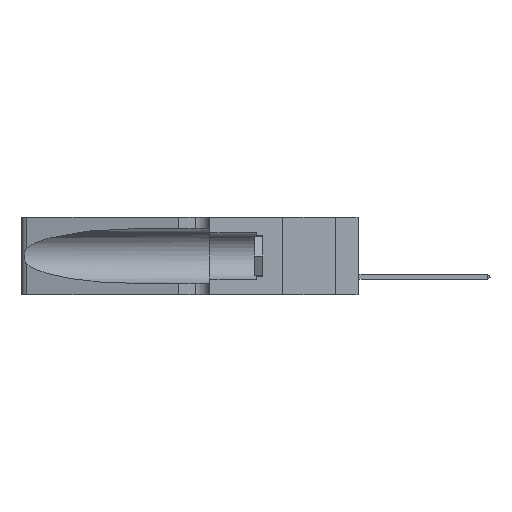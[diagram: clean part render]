
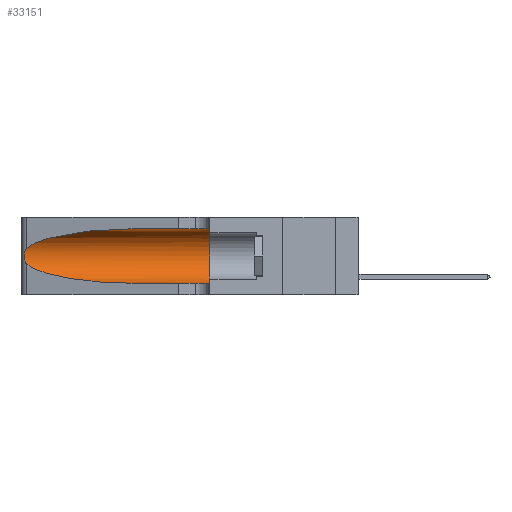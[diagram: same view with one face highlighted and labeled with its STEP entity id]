
A CAD part, left-side view. The second image highlights one B-rep face of the part: STEP entity #33151.
In plain terms, the highlighted cylindrical face has radius 3.308 mm (diameter 6.617 mm), a partial arc.
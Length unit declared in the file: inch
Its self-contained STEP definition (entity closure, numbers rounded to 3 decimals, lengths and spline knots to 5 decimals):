
#1242 = EDGE_CURVE ( 'NONE', #28191, #19521, #26771, .T. ) ;
#3250 = CARTESIAN_POINT ( 'NONE',  ( 0.1305, 0.72297, 0.05475 ) ) ;
#3714 = CARTESIAN_POINT ( 'NONE',  ( 0.25487, 1.22718, 0.14631 ) ) ;
#3749 = CIRCLE ( 'NONE', #8583, 0.13025 ) ;
#3908 = ORIENTED_EDGE ( 'NONE', *, *, #32514, .T. ) ;
#4390 =( BOUNDED_CURVE ( )  B_SPLINE_CURVE ( 3, ( #7320, #26133, #10004, #15291 ),
 .UNSPECIFIED., .F., .T. ) 
 B_SPLINE_CURVE_WITH_KNOTS ( ( 4, 4 ),
 ( 1.5708, 2.84003 ),
 .UNSPECIFIED. ) 
 CURVE ( )  GEOMETRIC_REPRESENTATION_ITEM ( )  RATIONAL_B_SPLINE_CURVE ( ( 1., 0.87, 0.87, 1. ) ) 
 REPRESENTATION_ITEM ( '' )  );
#5244 = EDGE_CURVE ( 'NONE', #26156, #19521, #3749, .T. ) ;
#5554 = VECTOR ( 'NONE', #18479, 39.37008 ) ;
#7320 = CARTESIAN_POINT ( 'NONE',  ( 0.1305, 0.72297, 0.31525 ) ) ;
#7625 = CARTESIAN_POINT ( 'NONE',  ( 0.25856, 1.23593, 0.16098 ) ) ;
#7730 = CARTESIAN_POINT ( 'NONE',  ( 0.25487, 1.22718, 0.14631 ) ) ;
#7751 = AXIS2_PLACEMENT_3D ( 'NONE', #30096, #32806, #21855 ) ;
#7841 = CARTESIAN_POINT ( 'NONE',  ( 0.25787, 1.23484, 0.2124 ) ) ;
#8583 = AXIS2_PLACEMENT_3D ( 'NONE', #32872, #8798, #27880 ) ;
#8798 = DIRECTION ( 'NONE',  ( 0., 1., 0. ) ) ;
#8917 = CARTESIAN_POINT ( 'NONE',  ( 0.1305, 0.72297, 0.31525 ) ) ;
#8945 = CARTESIAN_POINT ( 'NONE',  ( 0.1305, 0.35, 0.05475 ) ) ;
#9864 = VECTOR ( 'NONE', #13923, 39.37008 ) ;
#10004 = CARTESIAN_POINT ( 'NONE',  ( 0.2373, 1.15595, 0.28018 ) ) ;
#10185 = CARTESIAN_POINT ( 'NONE',  ( 0.26075, 1.23896, 0.178 ) ) ;
#10709 = VERTEX_POINT ( 'NONE', #32028 ) ;
#11398 = CARTESIAN_POINT ( 'NONE',  ( 0.25487, 1.22718, 0.14631 ) ) ;
#13778 = VERTEX_POINT ( 'NONE', #3714 ) ;
#13923 = DIRECTION ( 'NONE',  ( 0., -1., 0. ) ) ;
#14568 = ORIENTED_EDGE ( 'NONE', *, *, #1242, .T. ) ;
#14993 = CARTESIAN_POINT ( 'NONE',  ( 0.25487, 1.22718, 0.22369 ) ) ;
#15291 = CARTESIAN_POINT ( 'NONE',  ( 0.25487, 1.22718, 0.22369 ) ) ;
#15700 = CARTESIAN_POINT ( 'NONE',  ( 0.25639, 1.23186, 0.15144 ) ) ;
#15951 = CARTESIAN_POINT ( 'NONE',  ( 0.1305, 1.61858, 0.05475 ) ) ;
#16151 = EDGE_LOOP ( 'NONE', ( #28413, #30727, #3908, #14568, #30924, #21154 ) ) ;
#16345 = EDGE_CURVE ( 'NONE', #30201, #10709, #4390, .T. ) ;
#16499 = EDGE_CURVE ( 'NONE', #30201, #26156, #23954, .T. ) ;
#18227 = CARTESIAN_POINT ( 'NONE',  ( 0.26018, 1.23835, 0.19895 ) ) ;
#18479 = DIRECTION ( 'NONE',  ( 0., -1., 0. ) ) ;
#18659 = CARTESIAN_POINT ( 'NONE',  ( 0.26075, 1.23896, 0.19203 ) ) ;
#18864 =( BOUNDED_CURVE ( )  B_SPLINE_CURVE ( 3, ( #11398, #19206, #24425, #3250 ),
 .UNSPECIFIED., .F., .F. ) 
 B_SPLINE_CURVE_WITH_KNOTS ( ( 4, 4 ),
 ( 3.44316, 4.71239 ),
 .UNSPECIFIED. ) 
 CURVE ( )  GEOMETRIC_REPRESENTATION_ITEM ( )  RATIONAL_B_SPLINE_CURVE ( ( 1., 0.87, 0.87, 1. ) ) 
 REPRESENTATION_ITEM ( '' )  );
#18955 = FACE_OUTER_BOUND ( 'NONE', #16151, .T. ) ;
#18968 = CARTESIAN_POINT ( 'NONE',  ( 0.1305, 0.35, 0.31525 ) ) ;
#19206 = CARTESIAN_POINT ( 'NONE',  ( 0.2373, 1.15595, 0.08982 ) ) ;
#19521 = VERTEX_POINT ( 'NONE', #8945 ) ;
#20964 = CARTESIAN_POINT ( 'NONE',  ( 0.25639, 1.23184, 0.21858 ) ) ;
#21154 = ORIENTED_EDGE ( 'NONE', *, *, #16499, .F. ) ;
#21855 = DIRECTION ( 'NONE',  ( 0., 0., -1. ) ) ;
#23729 = EDGE_CURVE ( 'NONE', #10709, #13778, #25026, .T. ) ;
#23954 = LINE ( 'NONE', #24609, #9864 ) ;
#24425 = CARTESIAN_POINT ( 'NONE',  ( 0.18966, 0.96281, 0.05475 ) ) ;
#24609 = CARTESIAN_POINT ( 'NONE',  ( 0.1305, 1.61858, 0.31525 ) ) ;
#25026 = B_SPLINE_CURVE_WITH_KNOTS ( 'NONE', 3,
 ( #14993, #26197, #20964, #7841, #29206, #18227, #18659, #10185, #31468, #7625, #34383, #15700, #26412, #7730 ),
 .UNSPECIFIED., .F., .F.,
 ( 4, 2, 2, 2, 2, 2, 4 ),
 ( 0., 0.00027, 0.00053, 0.00107, 0.0016, 0.00187, 0.00214 ),
 .UNSPECIFIED. ) ;
#26133 = CARTESIAN_POINT ( 'NONE',  ( 0.18966, 0.96281, 0.31525 ) ) ;
#26156 = VERTEX_POINT ( 'NONE', #18968 ) ;
#26197 = CARTESIAN_POINT ( 'NONE',  ( 0.25555, 1.22994, 0.2215 ) ) ;
#26412 = CARTESIAN_POINT ( 'NONE',  ( 0.25555, 1.22993, 0.14849 ) ) ;
#26771 = LINE ( 'NONE', #15951, #5554 ) ;
#27880 = DIRECTION ( 'NONE',  ( 0., 0., 1. ) ) ;
#28191 = VERTEX_POINT ( 'NONE', #33598 ) ;
#28413 = ORIENTED_EDGE ( 'NONE', *, *, #16345, .T. ) ;
#29206 = CARTESIAN_POINT ( 'NONE',  ( 0.25854, 1.2359, 0.20912 ) ) ;
#30096 = CARTESIAN_POINT ( 'NONE',  ( 0.1305, 1.61858, 0.185 ) ) ;
#30201 = VERTEX_POINT ( 'NONE', #8917 ) ;
#30727 = ORIENTED_EDGE ( 'NONE', *, *, #23729, .T. ) ;
#30924 = ORIENTED_EDGE ( 'NONE', *, *, #5244, .F. ) ;
#31468 = CARTESIAN_POINT ( 'NONE',  ( 0.26017, 1.23833, 0.17102 ) ) ;
#31479 = CYLINDRICAL_SURFACE ( 'NONE', #7751, 0.13025 ) ;
#32028 = CARTESIAN_POINT ( 'NONE',  ( 0.25487, 1.22718, 0.22369 ) ) ;
#32514 = EDGE_CURVE ( 'NONE', #13778, #28191, #18864, .T. ) ;
#32806 = DIRECTION ( 'NONE',  ( 0., -1., 0. ) ) ;
#32872 = CARTESIAN_POINT ( 'NONE',  ( 0.1305, 0.35, 0.185 ) ) ;
#33151 = ADVANCED_FACE ( 'NONE', ( #18955 ), #31479, .F. ) ;
#33598 = CARTESIAN_POINT ( 'NONE',  ( 0.1305, 0.72297, 0.05475 ) ) ;
#34383 = CARTESIAN_POINT ( 'NONE',  ( 0.25789, 1.23486, 0.15765 ) ) ;
